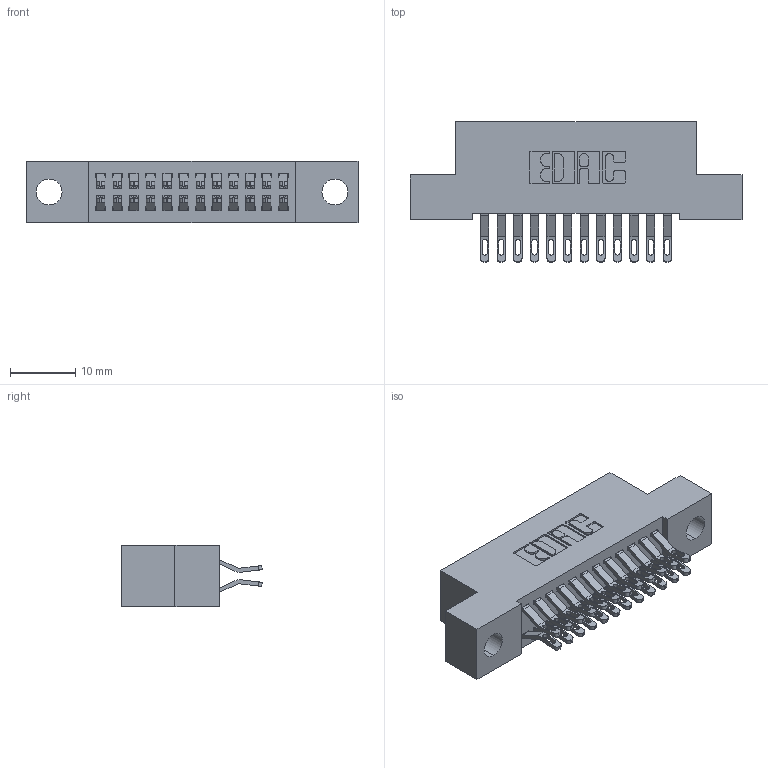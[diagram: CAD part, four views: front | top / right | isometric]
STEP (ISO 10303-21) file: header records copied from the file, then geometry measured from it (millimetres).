
FILE_DESCRIPTION (( 'STEP AP203' ), '1' );
FILE_NAME ('342-024-555-204.STEP', '2018-08-11T02:49:04', ( '' ), ( '' ), 'SwSTEP 2.0', 'SolidWorks 2016', '' );
FILE_SCHEMA (( 'CONFIG_CONTROL_DESIGN' ));
Length unit declared in the file: inch
Products named in the file (3): 342 Part_.156 TH; 345-292-001_555 Tail; 342-024-555-204
Assembly tree (25 placements, depth 2):
  342-024-555-204
    342 Part_.156 TH
    345-292-001_555 Tail  x24
Bounding box: 50.8 x 21.47 x 9.4 mm (x, y, z)
Volume: 4402 mm3; surface area: 6482.6 mm2
Topology: 25 solids, 25 shells, 1502 faces, 4691 edges, 3126 vertices
Faces by surface type: plane 882, cylinder 620
Entity records: 11797 total; most frequent: CARTESIAN_POINT 2024, ORIENTED_EDGE 1930, DIRECTION 1753, EDGE_CURVE 965, LINE 817, VECTOR 817, VERTEX_POINT 642, AXIS2_PLACEMENT_3D 468
